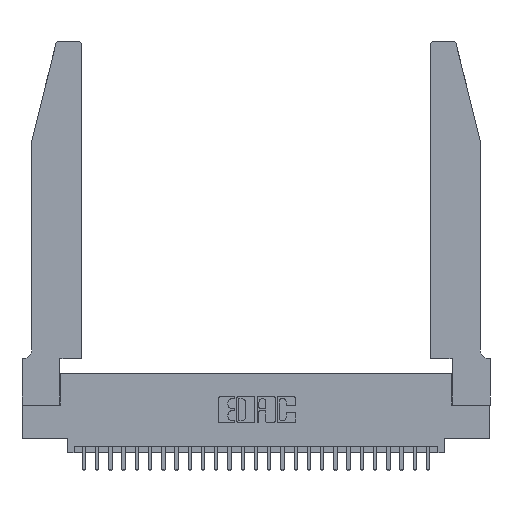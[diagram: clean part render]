
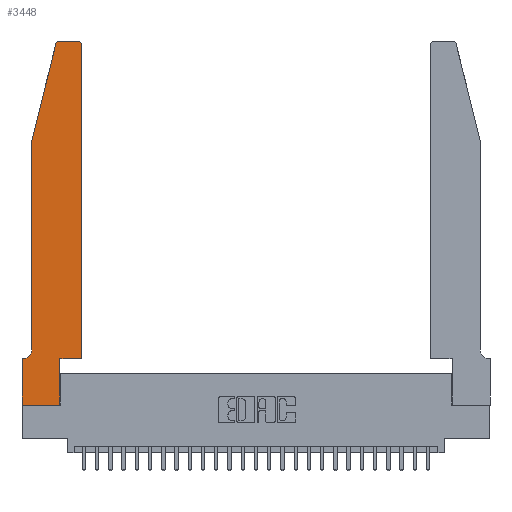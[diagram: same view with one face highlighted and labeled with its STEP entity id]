
A CAD part, top view. The second image highlights one B-rep face of the part: STEP entity #3448.
In plain terms, the highlighted planar face has unit normal (0, 0, 1).
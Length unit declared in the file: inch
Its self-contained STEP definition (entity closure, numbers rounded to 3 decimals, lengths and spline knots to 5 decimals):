
#190 = LINE ( 'NONE', #19734, #886 ) ;
#886 = VECTOR ( 'NONE', #6708, 39.37008 ) ;
#941 = EDGE_CURVE ( 'NONE', #22641, #6070, #24154, .T. ) ;
#1094 = AXIS2_PLACEMENT_3D ( 'NONE', #1791, #17144, #4024 ) ;
#1129 = VERTEX_POINT ( 'NONE', #4257 ) ;
#1396 = LINE ( 'NONE', #23979, #11761 ) ;
#1590 = CARTESIAN_POINT ( 'NONE',  ( 0., 0.35, 0.37 ) ) ;
#1791 = CARTESIAN_POINT ( 'NONE',  ( 0.284, 2.72, 0.37 ) ) ;
#2737 = CARTESIAN_POINT ( 'NONE',  ( 0.2605, 2.75, 0.37 ) ) ;
#2790 = VECTOR ( 'NONE', #13586, 39.37008 ) ;
#2886 = ORIENTED_EDGE ( 'NONE', *, *, #3210, .T. ) ;
#3210 = EDGE_CURVE ( 'NONE', #1129, #7014, #9987, .T. ) ;
#3448 = ADVANCED_FACE ( 'NONE', ( #5156 ), #25422, .T. ) ;
#3810 = LINE ( 'NONE', #2737, #26180 ) ;
#4024 = DIRECTION ( 'NONE',  ( 1., 0., 0. ) ) ;
#4142 = LINE ( 'NONE', #10249, #21507 ) ;
#4199 = VERTEX_POINT ( 'NONE', #6688 ) ;
#4238 = CARTESIAN_POINT ( 'NONE',  ( 0., 0.35, 0.37 ) ) ;
#4252 = VERTEX_POINT ( 'NONE', #8993 ) ;
#4257 = CARTESIAN_POINT ( 'NONE',  ( 0.0755, 0.42, 0.37 ) ) ;
#4714 = CARTESIAN_POINT ( 'NONE',  ( 0.4505, 0.35, 0.37 ) ) ;
#5156 = FACE_OUTER_BOUND ( 'NONE', #19318, .T. ) ;
#5273 = ORIENTED_EDGE ( 'NONE', *, *, #6524, .T. ) ;
#5335 = CIRCLE ( 'NONE', #1094, 0.03 ) ;
#5711 = CIRCLE ( 'NONE', #11098, 0.03 ) ;
#5841 = EDGE_CURVE ( 'NONE', #21498, #4252, #5711, .T. ) ;
#5915 = VECTOR ( 'NONE', #9326, 39.37008 ) ;
#6021 = VERTEX_POINT ( 'NONE', #17655 ) ;
#6070 = VERTEX_POINT ( 'NONE', #13293 ) ;
#6478 = EDGE_CURVE ( 'NONE', #6070, #21498, #13239, .T. ) ;
#6524 = EDGE_CURVE ( 'NONE', #26956, #27953, #5335, .T. ) ;
#6688 = CARTESIAN_POINT ( 'NONE',  ( 0.0755, 2., 0.37 ) ) ;
#6708 = DIRECTION ( 'NONE',  ( 0., -1., 0. ) ) ;
#6837 = CARTESIAN_POINT ( 'NONE',  ( 0.25487, 2.72718, 0.37 ) ) ;
#7014 = VERTEX_POINT ( 'NONE', #23373 ) ;
#7127 = CARTESIAN_POINT ( 'NONE',  ( 0., 0., 0.37 ) ) ;
#7546 = AXIS2_PLACEMENT_3D ( 'NONE', #1590, #8256, #23384 ) ;
#8256 = DIRECTION ( 'NONE',  ( 0., 0., 1. ) ) ;
#8368 = EDGE_CURVE ( 'NONE', #22822, #22641, #1396, .T. ) ;
#8627 = CARTESIAN_POINT ( 'NONE',  ( 0.0755, 2., 0.37 ) ) ;
#8993 = CARTESIAN_POINT ( 'NONE',  ( 0.4205, 2.75, 0.37 ) ) ;
#9326 = DIRECTION ( 'NONE',  ( 1., 0., 0. ) ) ;
#9423 = DIRECTION ( 'NONE',  ( 0., 0., -1. ) ) ;
#9512 = ORIENTED_EDGE ( 'NONE', *, *, #941, .T. ) ;
#9682 = CARTESIAN_POINT ( 'NONE',  ( 0.2865, 0., 0.37 ) ) ;
#9826 = ORIENTED_EDGE ( 'NONE', *, *, #6478, .T. ) ;
#9987 = CIRCLE ( 'NONE', #11054, 0.07 ) ;
#10127 = ORIENTED_EDGE ( 'NONE', *, *, #11297, .T. ) ;
#10249 = CARTESIAN_POINT ( 'NONE',  ( 0.0755, 0.35, 0.37 ) ) ;
#10386 = CARTESIAN_POINT ( 'NONE',  ( 0.4505, 0.35, 0.37 ) ) ;
#10755 = ORIENTED_EDGE ( 'NONE', *, *, #18941, .T. ) ;
#11054 = AXIS2_PLACEMENT_3D ( 'NONE', #22383, #9423, #24531 ) ;
#11098 = AXIS2_PLACEMENT_3D ( 'NONE', #24853, #11988, #26996 ) ;
#11297 = EDGE_CURVE ( 'NONE', #27349, #6021, #190, .T. ) ;
#11394 = CARTESIAN_POINT ( 'NONE',  ( 0.0755, 2., 0.37 ) ) ;
#11491 = CARTESIAN_POINT ( 'NONE',  ( 0.4505, 2.72, 0.37 ) ) ;
#11761 = VECTOR ( 'NONE', #17620, 39.37008 ) ;
#11988 = DIRECTION ( 'NONE',  ( 0., 0., 1. ) ) ;
#12550 = VECTOR ( 'NONE', #27587, 39.37008 ) ;
#13239 = LINE ( 'NONE', #10386, #12550 ) ;
#13293 = CARTESIAN_POINT ( 'NONE',  ( 0.4505, 0.35, 0.37 ) ) ;
#13586 = DIRECTION ( 'NONE',  ( -0.239, -0.971, 0. ) ) ;
#14631 = ORIENTED_EDGE ( 'NONE', *, *, #8368, .T. ) ;
#14814 = EDGE_CURVE ( 'NONE', #7014, #27349, #4142, .T. ) ;
#15871 = LINE ( 'NONE', #11394, #2790 ) ;
#17144 = DIRECTION ( 'NONE',  ( 0., 0., 1. ) ) ;
#17620 = DIRECTION ( 'NONE',  ( 0., 1., 0. ) ) ;
#17655 = CARTESIAN_POINT ( 'NONE',  ( 0., 0., 0.37 ) ) ;
#18206 = DIRECTION ( 'NONE',  ( 1., 0., 0. ) ) ;
#18941 = EDGE_CURVE ( 'NONE', #27953, #4199, #15871, .T. ) ;
#19180 = VECTOR ( 'NONE', #23746, 39.37008 ) ;
#19318 = EDGE_LOOP ( 'NONE', ( #26663, #5273, #10755, #28110, #2886, #28003, #10127, #21234, #14631, #9512, #9826, #23256 ) ) ;
#19734 = CARTESIAN_POINT ( 'NONE',  ( 0., 0., 0.37 ) ) ;
#21234 = ORIENTED_EDGE ( 'NONE', *, *, #22183, .T. ) ;
#21498 = VERTEX_POINT ( 'NONE', #11491 ) ;
#21507 = VECTOR ( 'NONE', #25302, 39.37008 ) ;
#22183 = EDGE_CURVE ( 'NONE', #6021, #22822, #23223, .T. ) ;
#22361 = DIRECTION ( 'NONE',  ( -1., 0., 0. ) ) ;
#22383 = CARTESIAN_POINT ( 'NONE',  ( 0.0055, 0.42, 0.37 ) ) ;
#22641 = VERTEX_POINT ( 'NONE', #24139 ) ;
#22736 = EDGE_CURVE ( 'NONE', #4252, #26956, #3810, .T. ) ;
#22822 = VERTEX_POINT ( 'NONE', #9682 ) ;
#23223 = LINE ( 'NONE', #7127, #5915 ) ;
#23256 = ORIENTED_EDGE ( 'NONE', *, *, #5841, .T. ) ;
#23373 = CARTESIAN_POINT ( 'NONE',  ( 0.0055, 0.35, 0.37 ) ) ;
#23384 = DIRECTION ( 'NONE',  ( 1., 0., 0. ) ) ;
#23480 = VECTOR ( 'NONE', #18206, 39.37008 ) ;
#23531 = EDGE_CURVE ( 'NONE', #4199, #1129, #24857, .T. ) ;
#23746 = DIRECTION ( 'NONE',  ( 0., -1., 0. ) ) ;
#23979 = CARTESIAN_POINT ( 'NONE',  ( 0.2865, 0.35, 0.37 ) ) ;
#24139 = CARTESIAN_POINT ( 'NONE',  ( 0.2865, 0.35, 0.37 ) ) ;
#24154 = LINE ( 'NONE', #4714, #23480 ) ;
#24531 = DIRECTION ( 'NONE',  ( -1., 0., 0. ) ) ;
#24656 = CARTESIAN_POINT ( 'NONE',  ( 0.284, 2.75, 0.37 ) ) ;
#24853 = CARTESIAN_POINT ( 'NONE',  ( 0.4205, 2.72, 0.37 ) ) ;
#24857 = LINE ( 'NONE', #8627, #19180 ) ;
#25302 = DIRECTION ( 'NONE',  ( -1., 0., 0. ) ) ;
#25422 = PLANE ( 'NONE',  #7546 ) ;
#26180 = VECTOR ( 'NONE', #22361, 39.37008 ) ;
#26663 = ORIENTED_EDGE ( 'NONE', *, *, #22736, .T. ) ;
#26956 = VERTEX_POINT ( 'NONE', #24656 ) ;
#26996 = DIRECTION ( 'NONE',  ( 1., 0., 0. ) ) ;
#27349 = VERTEX_POINT ( 'NONE', #4238 ) ;
#27587 = DIRECTION ( 'NONE',  ( 0., 1., 0. ) ) ;
#27953 = VERTEX_POINT ( 'NONE', #6837 ) ;
#28003 = ORIENTED_EDGE ( 'NONE', *, *, #14814, .T. ) ;
#28110 = ORIENTED_EDGE ( 'NONE', *, *, #23531, .T. ) ;
